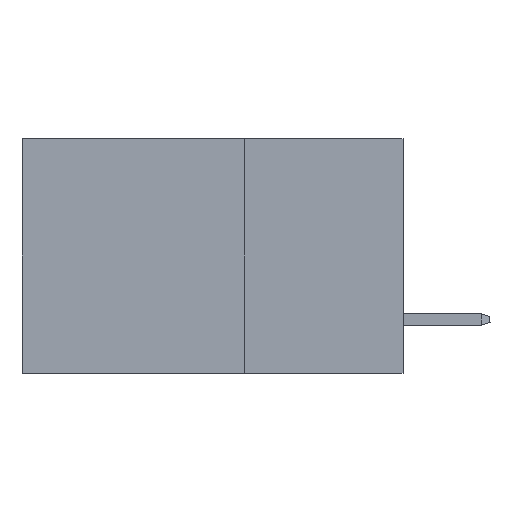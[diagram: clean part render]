
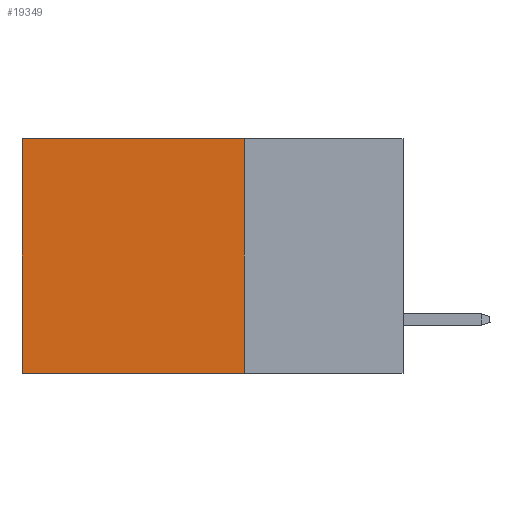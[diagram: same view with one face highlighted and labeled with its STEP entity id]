
A CAD part, left-side view. The second image highlights one B-rep face of the part: STEP entity #19349.
In plain terms, the highlighted planar face has unit normal (-1, 0, 0).
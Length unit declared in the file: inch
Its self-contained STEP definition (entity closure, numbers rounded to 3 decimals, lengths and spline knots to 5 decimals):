
#79 = PLANE ( 'NONE',  #12476 ) ;
#456 = CARTESIAN_POINT ( 'NONE',  ( 0.2875, 0.6, 0. ) ) ;
#2047 = LINE ( 'NONE', #9348, #14411 ) ;
#2483 = CARTESIAN_POINT ( 'NONE',  ( 0.2875, 0.25, -0.37 ) ) ;
#2543 = CARTESIAN_POINT ( 'NONE',  ( 0.2875, 0.25, 0. ) ) ;
#3698 = VERTEX_POINT ( 'NONE', #5501 ) ;
#3960 = EDGE_CURVE ( 'NONE', #20207, #9630, #16765, .T. ) ;
#4097 = DIRECTION ( 'NONE',  ( 0., 0., -1. ) ) ;
#4655 = DIRECTION ( 'NONE',  ( 0., 1., 0. ) ) ;
#5501 = CARTESIAN_POINT ( 'NONE',  ( 0.2875, 0.25, -0.37 ) ) ;
#6384 = DIRECTION ( 'NONE',  ( 0., 1., 0. ) ) ;
#6518 = VECTOR ( 'NONE', #21210, 39.37008 ) ;
#7461 = VECTOR ( 'NONE', #4655, 39.37008 ) ;
#8523 = CARTESIAN_POINT ( 'NONE',  ( 0.2875, 0.25, 0. ) ) ;
#8816 = CARTESIAN_POINT ( 'NONE',  ( 0.2875, 0.25, 0. ) ) ;
#9348 = CARTESIAN_POINT ( 'NONE',  ( 0.2875, 0.25, 0. ) ) ;
#9630 = VERTEX_POINT ( 'NONE', #19526 ) ;
#9651 = VECTOR ( 'NONE', #4097, 39.37008 ) ;
#9846 = DIRECTION ( 'NONE',  ( 0., 0., -1. ) ) ;
#10958 = EDGE_CURVE ( 'NONE', #14599, #20207, #2047, .T. ) ;
#11416 = DIRECTION ( 'NONE',  ( 1., 0., 0. ) ) ;
#12476 = AXIS2_PLACEMENT_3D ( 'NONE', #2543, #11416, #9846 ) ;
#13905 = EDGE_LOOP ( 'NONE', ( #19567, #16474, #22835, #20905 ) ) ;
#14079 = EDGE_CURVE ( 'NONE', #14599, #3698, #22880, .T. ) ;
#14411 = VECTOR ( 'NONE', #6384, 39.37008 ) ;
#14599 = VERTEX_POINT ( 'NONE', #8816 ) ;
#15219 = CARTESIAN_POINT ( 'NONE',  ( 0.2875, 0.6, 0. ) ) ;
#16474 = ORIENTED_EDGE ( 'NONE', *, *, #18659, .F. ) ;
#16765 = LINE ( 'NONE', #456, #9651 ) ;
#18096 = FACE_OUTER_BOUND ( 'NONE', #13905, .T. ) ;
#18659 = EDGE_CURVE ( 'NONE', #3698, #9630, #19117, .T. ) ;
#19117 = LINE ( 'NONE', #2483, #7461 ) ;
#19349 = ADVANCED_FACE ( 'NONE', ( #18096 ), #79, .F. ) ;
#19526 = CARTESIAN_POINT ( 'NONE',  ( 0.2875, 0.6, -0.37 ) ) ;
#19567 = ORIENTED_EDGE ( 'NONE', *, *, #3960, .T. ) ;
#20207 = VERTEX_POINT ( 'NONE', #15219 ) ;
#20905 = ORIENTED_EDGE ( 'NONE', *, *, #10958, .T. ) ;
#21210 = DIRECTION ( 'NONE',  ( 0., 0., -1. ) ) ;
#22835 = ORIENTED_EDGE ( 'NONE', *, *, #14079, .F. ) ;
#22880 = LINE ( 'NONE', #8523, #6518 ) ;
